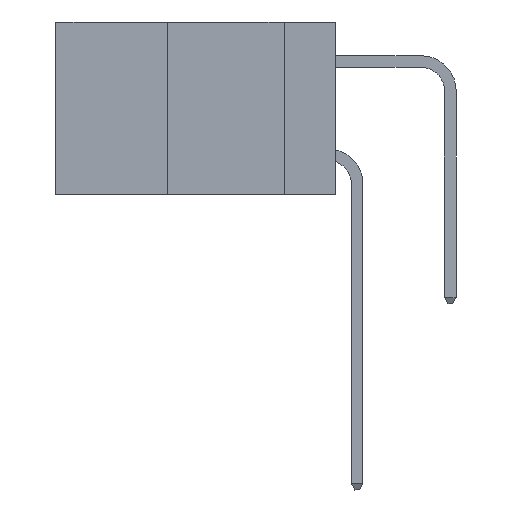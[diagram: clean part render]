
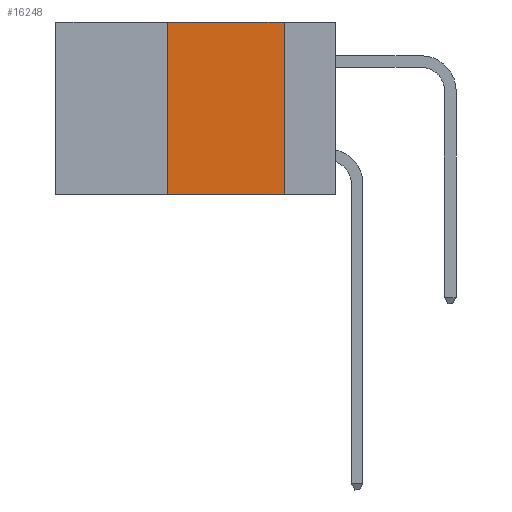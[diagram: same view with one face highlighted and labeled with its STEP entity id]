
A CAD part, left-side view. The second image highlights one B-rep face of the part: STEP entity #16248.
In plain terms, the highlighted planar face has unit normal (-1, 0, 0).
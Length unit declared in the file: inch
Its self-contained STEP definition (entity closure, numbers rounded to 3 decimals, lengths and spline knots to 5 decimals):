
#770 = FACE_OUTER_BOUND ( 'NONE', #1948, .T. ) ;
#1948 = EDGE_LOOP ( 'NONE', ( #16462, #15441, #1953, #3129 ) ) ;
#1953 = ORIENTED_EDGE ( 'NONE', *, *, #8400, .F. ) ;
#2313 = LINE ( 'NONE', #10159, #12900 ) ;
#2682 = PLANE ( 'NONE',  #16737 ) ;
#3129 = ORIENTED_EDGE ( 'NONE', *, *, #14611, .T. ) ;
#3366 = CARTESIAN_POINT ( 'NONE',  ( 0., 0.11, 0. ) ) ;
#4264 = DIRECTION ( 'NONE',  ( 0., -1., 0. ) ) ;
#4346 = EDGE_CURVE ( 'NONE', #11803, #15242, #14075, .T. ) ;
#4512 = CARTESIAN_POINT ( 'NONE',  ( 0., 0.36, 0. ) ) ;
#4608 = DIRECTION ( 'NONE',  ( 0., 0., -1. ) ) ;
#5541 = VECTOR ( 'NONE', #4264, 39.37008 ) ;
#6065 = CARTESIAN_POINT ( 'NONE',  ( 0., 0.11, -0.37 ) ) ;
#6558 = CARTESIAN_POINT ( 'NONE',  ( 0., 0.36, 0. ) ) ;
#7229 = CARTESIAN_POINT ( 'NONE',  ( 0., 0.11, 0. ) ) ;
#8400 = EDGE_CURVE ( 'NONE', #11837, #13740, #13293, .T. ) ;
#8533 = VECTOR ( 'NONE', #10076, 39.37008 ) ;
#8999 = CARTESIAN_POINT ( 'NONE',  ( 0., 0.36, -0.37 ) ) ;
#10076 = DIRECTION ( 'NONE',  ( 0., 0., 1. ) ) ;
#10134 = CARTESIAN_POINT ( 'NONE',  ( 0., 0.6, -0.37 ) ) ;
#10159 = CARTESIAN_POINT ( 'NONE',  ( 0., 0.6, 0. ) ) ;
#10339 = DIRECTION ( 'NONE',  ( 0., -1., 0. ) ) ;
#10388 = LINE ( 'NONE', #10134, #5541 ) ;
#10420 = VECTOR ( 'NONE', #4608, 39.37008 ) ;
#10852 = CARTESIAN_POINT ( 'NONE',  ( 0., 0.6, 0. ) ) ;
#11803 = VERTEX_POINT ( 'NONE', #7229 ) ;
#11837 = VERTEX_POINT ( 'NONE', #8999 ) ;
#12560 = EDGE_CURVE ( 'NONE', #13740, #11803, #2313, .T. ) ;
#12900 = VECTOR ( 'NONE', #10339, 39.37008 ) ;
#13293 = LINE ( 'NONE', #4512, #8533 ) ;
#13740 = VERTEX_POINT ( 'NONE', #6558 ) ;
#14075 = LINE ( 'NONE', #3366, #10420 ) ;
#14611 = EDGE_CURVE ( 'NONE', #11837, #15242, #10388, .T. ) ;
#15069 = DIRECTION ( 'NONE',  ( 0., 0., -1. ) ) ;
#15242 = VERTEX_POINT ( 'NONE', #6065 ) ;
#15441 = ORIENTED_EDGE ( 'NONE', *, *, #12560, .F. ) ;
#16248 = ADVANCED_FACE ( 'NONE', ( #770 ), #2682, .F. ) ;
#16354 = DIRECTION ( 'NONE',  ( 1., 0., 0. ) ) ;
#16462 = ORIENTED_EDGE ( 'NONE', *, *, #4346, .F. ) ;
#16737 = AXIS2_PLACEMENT_3D ( 'NONE', #10852, #16354, #15069 ) ;
